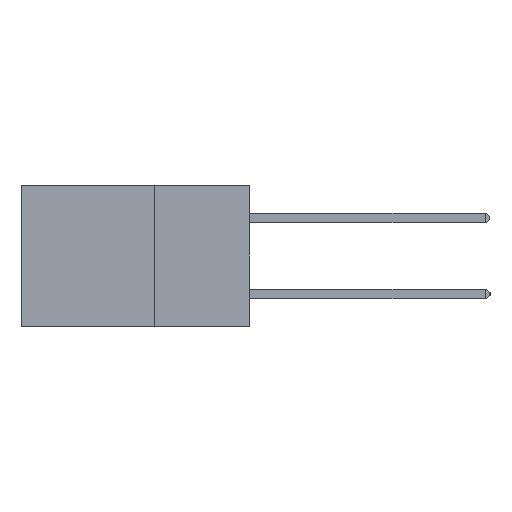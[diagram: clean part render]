
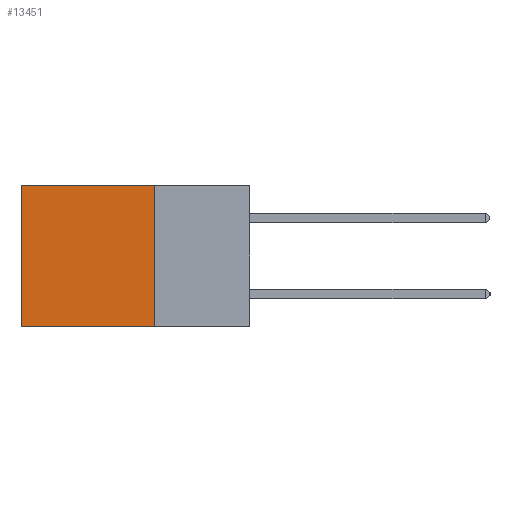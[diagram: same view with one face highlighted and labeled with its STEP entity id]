
A CAD part, left-side view. The second image highlights one B-rep face of the part: STEP entity #13451.
In plain terms, the highlighted planar face has unit normal (-1, 0, 0).
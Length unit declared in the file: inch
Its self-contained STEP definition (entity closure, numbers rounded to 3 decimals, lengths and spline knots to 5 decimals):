
#17 = VECTOR ( 'NONE', #1934, 39.37008 ) ;
#204 = CARTESIAN_POINT ( 'NONE',  ( 0.2875, 0.25, -0.37 ) ) ;
#1826 = ORIENTED_EDGE ( 'NONE', *, *, #4646, .F. ) ;
#1934 = DIRECTION ( 'NONE',  ( 0., 1., 0. ) ) ;
#2078 = ORIENTED_EDGE ( 'NONE', *, *, #6005, .F. ) ;
#3188 = VERTEX_POINT ( 'NONE', #5404 ) ;
#3800 = DIRECTION ( 'NONE',  ( 0., 0., -1. ) ) ;
#4001 = DIRECTION ( 'NONE',  ( 0., 0., -1. ) ) ;
#4311 = AXIS2_PLACEMENT_3D ( 'NONE', #7259, #19040, #8999 ) ;
#4646 = EDGE_CURVE ( 'NONE', #7903, #9173, #9637, .T. ) ;
#5404 = CARTESIAN_POINT ( 'NONE',  ( 0.2875, 0.6, 0. ) ) ;
#5939 = EDGE_LOOP ( 'NONE', ( #19850, #1826, #2078, #19974 ) ) ;
#6005 = EDGE_CURVE ( 'NONE', #15011, #7903, #12512, .T. ) ;
#6244 = VECTOR ( 'NONE', #13507, 39.37008 ) ;
#6682 = CARTESIAN_POINT ( 'NONE',  ( 0.2875, 0.25, 0. ) ) ;
#7104 = CARTESIAN_POINT ( 'NONE',  ( 0.2875, 0.6, 0. ) ) ;
#7193 = EDGE_CURVE ( 'NONE', #3188, #9173, #10055, .T. ) ;
#7259 = CARTESIAN_POINT ( 'NONE',  ( 0.2875, 0.25, 0. ) ) ;
#7903 = VERTEX_POINT ( 'NONE', #19356 ) ;
#8215 = EDGE_CURVE ( 'NONE', #15011, #3188, #20189, .T. ) ;
#8999 = DIRECTION ( 'NONE',  ( 0., 0., -1. ) ) ;
#9173 = VERTEX_POINT ( 'NONE', #20813 ) ;
#9637 = LINE ( 'NONE', #204, #17 ) ;
#10055 = LINE ( 'NONE', #7104, #14035 ) ;
#12512 = LINE ( 'NONE', #14240, #16444 ) ;
#13451 = ADVANCED_FACE ( 'NONE', ( #16382 ), #17385, .F. ) ;
#13507 = DIRECTION ( 'NONE',  ( 0., 1., 0. ) ) ;
#14035 = VECTOR ( 'NONE', #3800, 39.37008 ) ;
#14240 = CARTESIAN_POINT ( 'NONE',  ( 0.2875, 0.25, 0. ) ) ;
#15011 = VERTEX_POINT ( 'NONE', #6682 ) ;
#15157 = CARTESIAN_POINT ( 'NONE',  ( 0.2875, 0.25, 0. ) ) ;
#16382 = FACE_OUTER_BOUND ( 'NONE', #5939, .T. ) ;
#16444 = VECTOR ( 'NONE', #4001, 39.37008 ) ;
#17385 = PLANE ( 'NONE',  #4311 ) ;
#19040 = DIRECTION ( 'NONE',  ( 1., 0., 0. ) ) ;
#19356 = CARTESIAN_POINT ( 'NONE',  ( 0.2875, 0.25, -0.37 ) ) ;
#19850 = ORIENTED_EDGE ( 'NONE', *, *, #7193, .T. ) ;
#19974 = ORIENTED_EDGE ( 'NONE', *, *, #8215, .T. ) ;
#20189 = LINE ( 'NONE', #15157, #6244 ) ;
#20813 = CARTESIAN_POINT ( 'NONE',  ( 0.2875, 0.6, -0.37 ) ) ;
